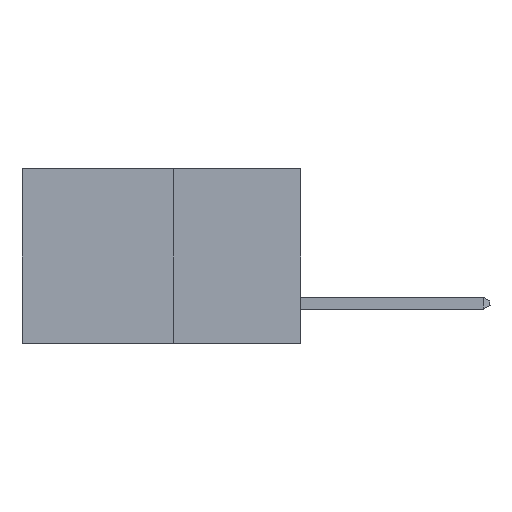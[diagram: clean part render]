
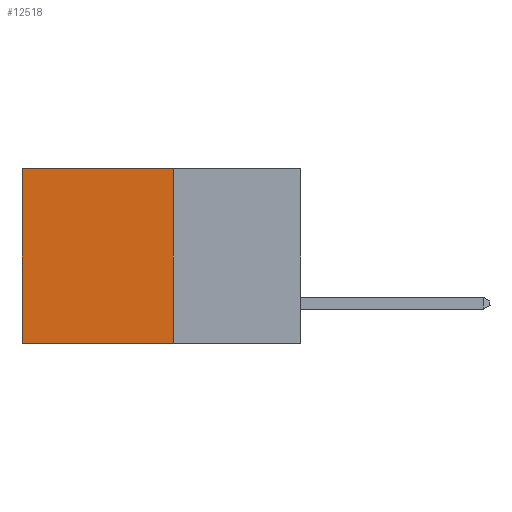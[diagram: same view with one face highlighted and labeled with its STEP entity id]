
A CAD part, left-side view. The second image highlights one B-rep face of the part: STEP entity #12518.
In plain terms, the highlighted planar face has unit normal (-1, 0, 0).
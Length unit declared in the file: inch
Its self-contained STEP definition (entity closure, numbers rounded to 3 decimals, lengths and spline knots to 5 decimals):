
#376 = EDGE_CURVE ( 'NONE', #21116, #491, #17047, .T. ) ;
#491 = VERTEX_POINT ( 'NONE', #1886 ) ;
#1886 = CARTESIAN_POINT ( 'NONE',  ( 0.277, 0.59, -0.37 ) ) ;
#2373 = CARTESIAN_POINT ( 'NONE',  ( 0.277, 0.27, -0.37 ) ) ;
#3334 = AXIS2_PLACEMENT_3D ( 'NONE', #2373, #15521, #4344 ) ;
#4344 = DIRECTION ( 'NONE',  ( 0., 0., -1. ) ) ;
#4608 = DIRECTION ( 'NONE',  ( 0., 1., 0. ) ) ;
#5808 = CARTESIAN_POINT ( 'NONE',  ( 0.277, 0.27, 0. ) ) ;
#6075 = ORIENTED_EDGE ( 'NONE', *, *, #23697, .T. ) ;
#7190 = VECTOR ( 'NONE', #16534, 39.37008 ) ;
#7207 = VECTOR ( 'NONE', #18925, 39.37008 ) ;
#7513 = DIRECTION ( 'NONE',  ( 0., 0., -1. ) ) ;
#9695 = ORIENTED_EDGE ( 'NONE', *, *, #376, .F. ) ;
#10600 = LINE ( 'NONE', #17614, #11177 ) ;
#11177 = VECTOR ( 'NONE', #4608, 39.37008 ) ;
#12518 = ADVANCED_FACE ( 'NONE', ( #15755 ), #13686, .F. ) ;
#13429 = CARTESIAN_POINT ( 'NONE',  ( 0.277, 0.59, -0.37 ) ) ;
#13686 = PLANE ( 'NONE',  #3334 ) ;
#14440 = CARTESIAN_POINT ( 'NONE',  ( 0.277, 0.59, 0. ) ) ;
#15193 = VECTOR ( 'NONE', #7513, 39.37008 ) ;
#15448 = EDGE_LOOP ( 'NONE', ( #20403, #9695, #20342, #6075 ) ) ;
#15494 = CARTESIAN_POINT ( 'NONE',  ( 0.277, 0.27, -0.37 ) ) ;
#15521 = DIRECTION ( 'NONE',  ( 1., 0., 0. ) ) ;
#15755 = FACE_OUTER_BOUND ( 'NONE', #15448, .T. ) ;
#15759 = LINE ( 'NONE', #22198, #15193 ) ;
#16534 = DIRECTION ( 'NONE',  ( 0., 1., 0. ) ) ;
#17047 = LINE ( 'NONE', #21908, #7190 ) ;
#17614 = CARTESIAN_POINT ( 'NONE',  ( 0.277, 0.27, 0. ) ) ;
#17734 = EDGE_CURVE ( 'NONE', #20635, #21116, #15759, .T. ) ;
#18925 = DIRECTION ( 'NONE',  ( 0., 0., -1. ) ) ;
#20342 = ORIENTED_EDGE ( 'NONE', *, *, #17734, .F. ) ;
#20403 = ORIENTED_EDGE ( 'NONE', *, *, #21016, .T. ) ;
#20635 = VERTEX_POINT ( 'NONE', #5808 ) ;
#21016 = EDGE_CURVE ( 'NONE', #22588, #491, #21867, .T. ) ;
#21116 = VERTEX_POINT ( 'NONE', #15494 ) ;
#21867 = LINE ( 'NONE', #13429, #7207 ) ;
#21908 = CARTESIAN_POINT ( 'NONE',  ( 0.277, 0.27, -0.37 ) ) ;
#22198 = CARTESIAN_POINT ( 'NONE',  ( 0.277, 0.27, -0.37 ) ) ;
#22588 = VERTEX_POINT ( 'NONE', #14440 ) ;
#23697 = EDGE_CURVE ( 'NONE', #20635, #22588, #10600, .T. ) ;
